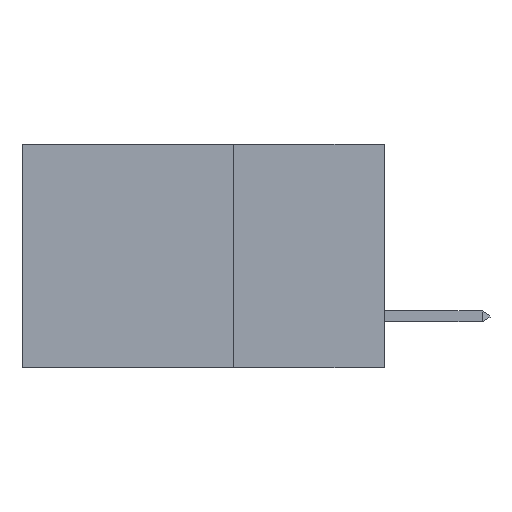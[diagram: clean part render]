
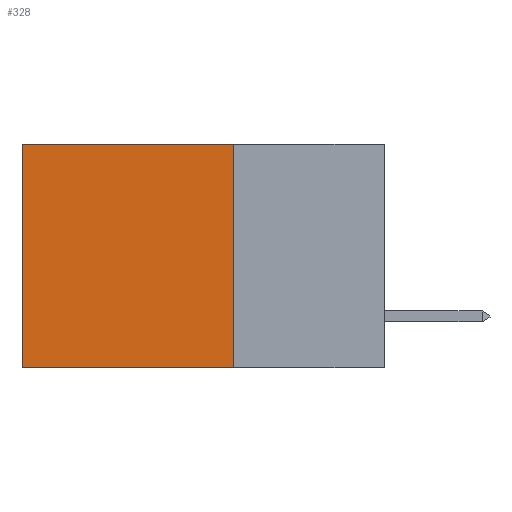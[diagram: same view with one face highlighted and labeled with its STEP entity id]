
A CAD part, left-side view. The second image highlights one B-rep face of the part: STEP entity #328.
In plain terms, the highlighted planar face has unit normal (-1, 0, 0).
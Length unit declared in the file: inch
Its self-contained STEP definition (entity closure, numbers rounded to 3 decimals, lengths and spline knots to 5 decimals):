
#197 = VERTEX_POINT ( 'NONE', #7328 ) ;
#328 = ADVANCED_FACE ( 'NONE', ( #6373 ), #10917, .F. ) ;
#939 = EDGE_CURVE ( 'NONE', #4884, #11349, #10649, .T. ) ;
#1244 = LINE ( 'NONE', #11724, #5945 ) ;
#1728 = VERTEX_POINT ( 'NONE', #2222 ) ;
#1996 = LINE ( 'NONE', #6214, #11290 ) ;
#2222 = CARTESIAN_POINT ( 'NONE',  ( 0.2875, 0.6, 0. ) ) ;
#2327 = CARTESIAN_POINT ( 'NONE',  ( 0.2875, 0.25, 0. ) ) ;
#3144 = CARTESIAN_POINT ( 'NONE',  ( 0.2875, 0.25, -0.37 ) ) ;
#3440 = DIRECTION ( 'NONE',  ( 0., 0., -1. ) ) ;
#4880 = AXIS2_PLACEMENT_3D ( 'NONE', #5171, #11116, #11549 ) ;
#4883 = VECTOR ( 'NONE', #10312, 39.37008 ) ;
#4884 = VERTEX_POINT ( 'NONE', #2327 ) ;
#5171 = CARTESIAN_POINT ( 'NONE',  ( 0.2875, 0.25, 0. ) ) ;
#5945 = VECTOR ( 'NONE', #8258, 39.37008 ) ;
#6214 = CARTESIAN_POINT ( 'NONE',  ( 0.2875, 0.6, 0. ) ) ;
#6225 = VECTOR ( 'NONE', #9819, 39.37008 ) ;
#6373 = FACE_OUTER_BOUND ( 'NONE', #6957, .T. ) ;
#6895 = EDGE_CURVE ( 'NONE', #4884, #1728, #1244, .T. ) ;
#6957 = EDGE_LOOP ( 'NONE', ( #7918, #8515, #9656, #11750 ) ) ;
#7328 = CARTESIAN_POINT ( 'NONE',  ( 0.2875, 0.6, -0.37 ) ) ;
#7718 = CARTESIAN_POINT ( 'NONE',  ( 0.2875, 0.25, -0.37 ) ) ;
#7854 = LINE ( 'NONE', #3144, #4883 ) ;
#7918 = ORIENTED_EDGE ( 'NONE', *, *, #8089, .T. ) ;
#8089 = EDGE_CURVE ( 'NONE', #1728, #197, #1996, .T. ) ;
#8258 = DIRECTION ( 'NONE',  ( 0., 1., 0. ) ) ;
#8515 = ORIENTED_EDGE ( 'NONE', *, *, #10565, .F. ) ;
#9656 = ORIENTED_EDGE ( 'NONE', *, *, #939, .F. ) ;
#9819 = DIRECTION ( 'NONE',  ( 0., 0., -1. ) ) ;
#9830 = CARTESIAN_POINT ( 'NONE',  ( 0.2875, 0.25, 0. ) ) ;
#10312 = DIRECTION ( 'NONE',  ( 0., 1., 0. ) ) ;
#10565 = EDGE_CURVE ( 'NONE', #11349, #197, #7854, .T. ) ;
#10649 = LINE ( 'NONE', #9830, #6225 ) ;
#10917 = PLANE ( 'NONE',  #4880 ) ;
#11116 = DIRECTION ( 'NONE',  ( 1., 0., 0. ) ) ;
#11290 = VECTOR ( 'NONE', #3440, 39.37008 ) ;
#11349 = VERTEX_POINT ( 'NONE', #7718 ) ;
#11549 = DIRECTION ( 'NONE',  ( 0., 0., -1. ) ) ;
#11724 = CARTESIAN_POINT ( 'NONE',  ( 0.2875, 0.25, 0. ) ) ;
#11750 = ORIENTED_EDGE ( 'NONE', *, *, #6895, .T. ) ;
